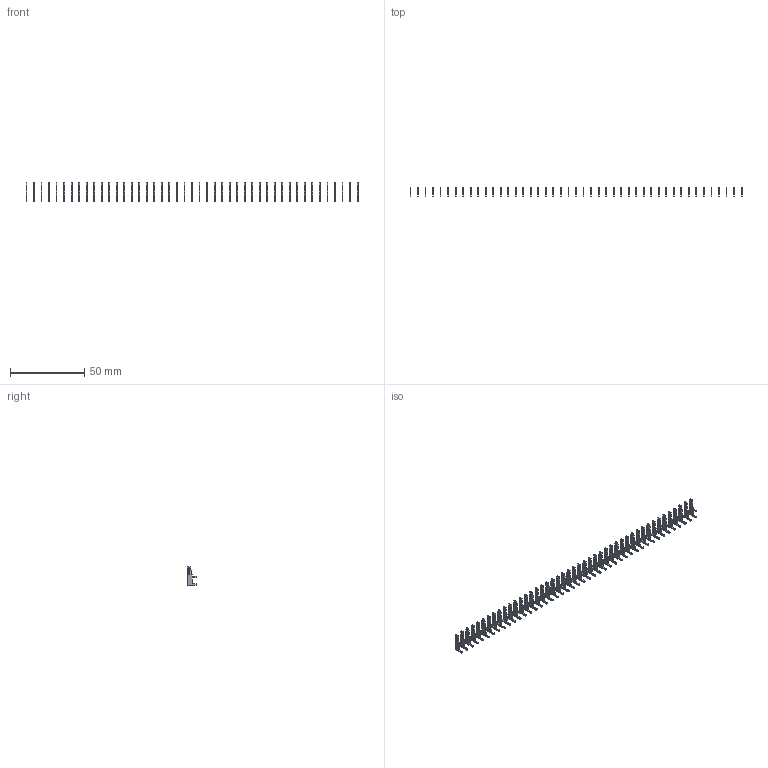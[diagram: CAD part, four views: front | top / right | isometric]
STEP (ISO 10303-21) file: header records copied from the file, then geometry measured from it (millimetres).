
FILE_DESCRIPTION (( 'STEP AP203' ), '1' );
FILE_NAME ('105-045-203-200.STEP', '2020-08-29T23:48:24', ( '' ), ( '' ), 'SwSTEP 2.0', 'SolidWorks 2020', '' );
FILE_SCHEMA (( 'CONFIG_CONTROL_DESIGN' ));
Length unit declared in the file: inch
Products named in the file (2): 105-045-203-200; 100-290-001_100-290-203
Assembly tree (45 placements, depth 2):
  105-045-203-200
    100-290-001_100-290-203  x45
Bounding box: 224.12 x 6.53 x 12.7 mm (x, y, z)
Volume: 1136.1 mm3; surface area: 5207.4 mm2
Topology: 45 solids, 45 shells, 1260 faces, 3510 edges, 2340 vertices
Faces by surface type: plane 945, cylinder 315
Entity records: 2504 total; most frequent: DIRECTION 240, CARTESIAN_POINT 218, ORIENTED_EDGE 156, LOCAL_TIME 100, COORDINATED_UNIVERSAL_TIME_OFFSET 100, CALENDAR_DATE 100, DATE_AND_TIME 100, AXIS2_PLACEMENT_3D 90
